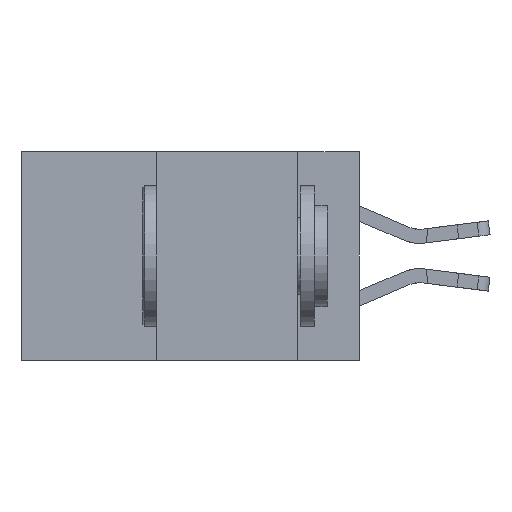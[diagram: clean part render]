
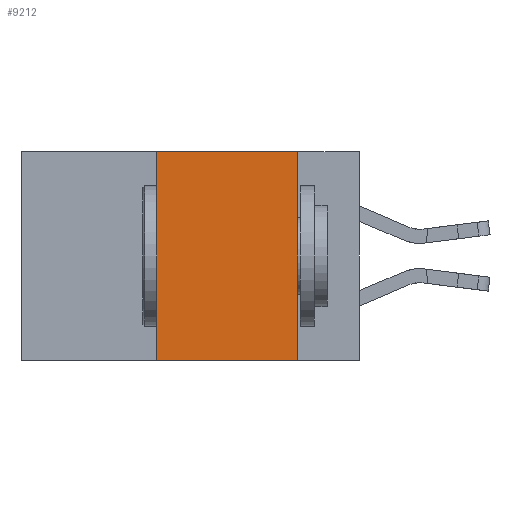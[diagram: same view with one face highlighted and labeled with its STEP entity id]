
A CAD part, left-side view. The second image highlights one B-rep face of the part: STEP entity #9212.
In plain terms, the highlighted planar face has unit normal (-1, 0, 0).
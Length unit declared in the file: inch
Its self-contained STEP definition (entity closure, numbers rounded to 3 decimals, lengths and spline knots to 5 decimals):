
#806 = DIRECTION ( 'NONE',  ( 0., 0., 1. ) ) ;
#878 = CARTESIAN_POINT ( 'NONE',  ( 0., 0.11, -0.37 ) ) ;
#888 = ORIENTED_EDGE ( 'NONE', *, *, #1397, .F. ) ;
#1397 = EDGE_CURVE ( 'NONE', #13110, #16268, #12768, .T. ) ;
#1521 = ORIENTED_EDGE ( 'NONE', *, *, #2959, .F. ) ;
#1655 = CARTESIAN_POINT ( 'NONE',  ( 0., 0.11, 0. ) ) ;
#1953 = EDGE_LOOP ( 'NONE', ( #10749, #1521, #888, #10226 ) ) ;
#2959 = EDGE_CURVE ( 'NONE', #16268, #6604, #5655, .T. ) ;
#3221 = DIRECTION ( 'NONE',  ( 0., 0., -1. ) ) ;
#3720 = DIRECTION ( 'NONE',  ( 0., -1., 0. ) ) ;
#4018 = VECTOR ( 'NONE', #806, 39.37008 ) ;
#4830 = CARTESIAN_POINT ( 'NONE',  ( 0., 0.36, 0. ) ) ;
#4878 = LINE ( 'NONE', #7784, #10041 ) ;
#5655 = LINE ( 'NONE', #8891, #6970 ) ;
#6109 = CARTESIAN_POINT ( 'NONE',  ( 0., 0.6, 0. ) ) ;
#6604 = VERTEX_POINT ( 'NONE', #8813 ) ;
#6970 = VECTOR ( 'NONE', #13109, 39.37008 ) ;
#7321 = DIRECTION ( 'NONE',  ( 1., 0., 0. ) ) ;
#7552 = PLANE ( 'NONE',  #13927 ) ;
#7784 = CARTESIAN_POINT ( 'NONE',  ( 0., 0.6, -0.37 ) ) ;
#8102 = EDGE_CURVE ( 'NONE', #13110, #12182, #4878, .T. ) ;
#8813 = CARTESIAN_POINT ( 'NONE',  ( 0., 0.11, 0. ) ) ;
#8891 = CARTESIAN_POINT ( 'NONE',  ( 0., 0.6, 0. ) ) ;
#9212 = ADVANCED_FACE ( 'NONE', ( #9578 ), #7552, .F. ) ;
#9578 = FACE_OUTER_BOUND ( 'NONE', #1953, .T. ) ;
#9837 = VECTOR ( 'NONE', #3221, 39.37008 ) ;
#10041 = VECTOR ( 'NONE', #3720, 39.37008 ) ;
#10226 = ORIENTED_EDGE ( 'NONE', *, *, #8102, .T. ) ;
#10749 = ORIENTED_EDGE ( 'NONE', *, *, #16031, .F. ) ;
#12182 = VERTEX_POINT ( 'NONE', #878 ) ;
#12768 = LINE ( 'NONE', #15806, #4018 ) ;
#13109 = DIRECTION ( 'NONE',  ( 0., -1., 0. ) ) ;
#13110 = VERTEX_POINT ( 'NONE', #17465 ) ;
#13927 = AXIS2_PLACEMENT_3D ( 'NONE', #6109, #7321, #17185 ) ;
#15806 = CARTESIAN_POINT ( 'NONE',  ( 0., 0.36, 0. ) ) ;
#16031 = EDGE_CURVE ( 'NONE', #6604, #12182, #16354, .T. ) ;
#16268 = VERTEX_POINT ( 'NONE', #4830 ) ;
#16354 = LINE ( 'NONE', #1655, #9837 ) ;
#17185 = DIRECTION ( 'NONE',  ( 0., 0., -1. ) ) ;
#17465 = CARTESIAN_POINT ( 'NONE',  ( 0., 0.36, -0.37 ) ) ;
